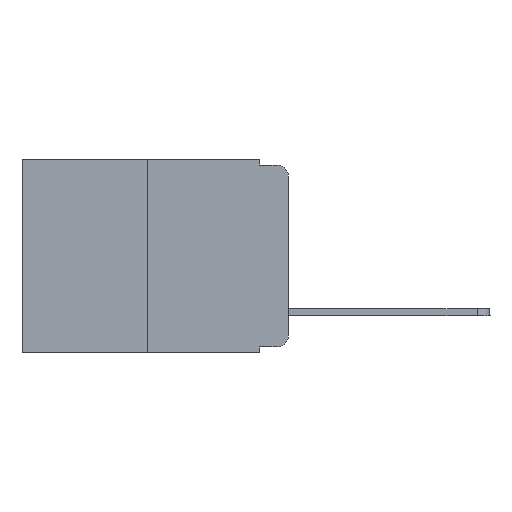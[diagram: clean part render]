
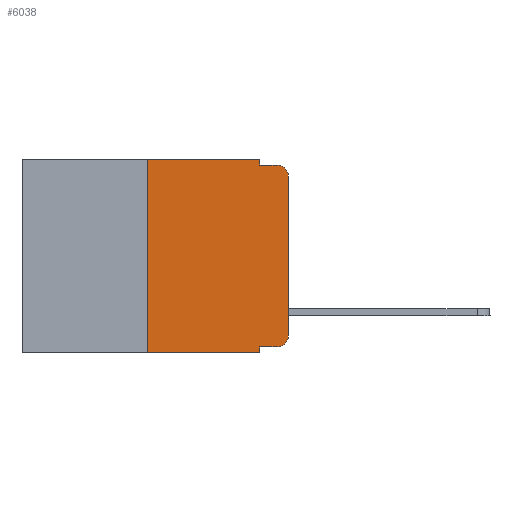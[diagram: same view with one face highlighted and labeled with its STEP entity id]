
A CAD part, left-side view. The second image highlights one B-rep face of the part: STEP entity #6038.
In plain terms, the highlighted planar face has unit normal (-1, 0, 0).
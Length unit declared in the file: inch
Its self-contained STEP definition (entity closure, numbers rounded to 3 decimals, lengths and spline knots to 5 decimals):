
#55 = LINE ( 'NONE', #207, #665 ) ;
#207 = CARTESIAN_POINT ( 'NONE',  ( 0., 0.051, 0. ) ) ;
#636 = CARTESIAN_POINT ( 'NONE',  ( 0., 0.25, 0. ) ) ;
#665 = VECTOR ( 'NONE', #2945, 39.37008 ) ;
#718 = DIRECTION ( 'NONE',  ( 0., 0., -1. ) ) ;
#817 = FACE_OUTER_BOUND ( 'NONE', #9570, .T. ) ;
#1017 = LINE ( 'NONE', #8204, #3437 ) ;
#1083 = VERTEX_POINT ( 'NONE', #6761 ) ;
#1377 = VECTOR ( 'NONE', #4258, 39.37008 ) ;
#1836 = DIRECTION ( 'NONE',  ( 0., 0., 1. ) ) ;
#1902 = DIRECTION ( 'NONE',  ( -1., 0., 0. ) ) ;
#1961 = EDGE_CURVE ( 'NONE', #9466, #3593, #12569, .T. ) ;
#2241 = ORIENTED_EDGE ( 'NONE', *, *, #13713, .T. ) ;
#2473 = EDGE_CURVE ( 'NONE', #8637, #9645, #10132, .T. ) ;
#2530 = CARTESIAN_POINT ( 'NONE',  ( 0., 0.051, -0.333 ) ) ;
#2765 = LINE ( 'NONE', #5359, #1377 ) ;
#2816 = CARTESIAN_POINT ( 'NONE',  ( 0., 0., -0.313 ) ) ;
#2838 = DIRECTION ( 'NONE',  ( 0., -1., 0. ) ) ;
#2945 = DIRECTION ( 'NONE',  ( 0., 0., -1. ) ) ;
#3437 = VECTOR ( 'NONE', #1836, 39.37008 ) ;
#3593 = VERTEX_POINT ( 'NONE', #9325 ) ;
#3836 = DIRECTION ( 'NONE',  ( -1., 0., 0. ) ) ;
#3956 = CIRCLE ( 'NONE', #6671, 0.02 ) ;
#4243 = AXIS2_PLACEMENT_3D ( 'NONE', #8437, #15005, #7209 ) ;
#4258 = DIRECTION ( 'NONE',  ( 0., -1., 0. ) ) ;
#4588 = CARTESIAN_POINT ( 'NONE',  ( 0., 0.25, -0.343 ) ) ;
#4940 = CARTESIAN_POINT ( 'NONE',  ( 0., 0.473, 0. ) ) ;
#5207 = CARTESIAN_POINT ( 'NONE',  ( 0., 0.051, -0.01 ) ) ;
#5359 = CARTESIAN_POINT ( 'NONE',  ( 0., 0.473, -0.343 ) ) ;
#5781 = EDGE_CURVE ( 'NONE', #1083, #15690, #7838, .T. ) ;
#5980 = EDGE_CURVE ( 'NONE', #6681, #8637, #1017, .T. ) ;
#6038 = ADVANCED_FACE ( 'NONE', ( #817 ), #14897, .F. ) ;
#6141 = LINE ( 'NONE', #14799, #15183 ) ;
#6408 = ORIENTED_EDGE ( 'NONE', *, *, #5980, .F. ) ;
#6595 = CARTESIAN_POINT ( 'NONE',  ( 0., 0.051, -0.01 ) ) ;
#6671 = AXIS2_PLACEMENT_3D ( 'NONE', #10953, #3836, #16038 ) ;
#6681 = VERTEX_POINT ( 'NONE', #4588 ) ;
#6761 = CARTESIAN_POINT ( 'NONE',  ( 0., 0.051, -0.333 ) ) ;
#6829 = VECTOR ( 'NONE', #12803, 39.37008 ) ;
#6850 = CIRCLE ( 'NONE', #14846, 0.02 ) ;
#6898 = VERTEX_POINT ( 'NONE', #5207 ) ;
#7050 = CARTESIAN_POINT ( 'NONE',  ( 0., 0.02, -0.03 ) ) ;
#7209 = DIRECTION ( 'NONE',  ( 0., 0., -1. ) ) ;
#7406 = EDGE_CURVE ( 'NONE', #6681, #9851, #2765, .T. ) ;
#7838 = LINE ( 'NONE', #2530, #6829 ) ;
#7950 = VECTOR ( 'NONE', #15920, 39.37008 ) ;
#8204 = CARTESIAN_POINT ( 'NONE',  ( 0., 0.25, 0. ) ) ;
#8404 = EDGE_CURVE ( 'NONE', #1083, #9851, #6141, .T. ) ;
#8436 = ORIENTED_EDGE ( 'NONE', *, *, #11366, .F. ) ;
#8437 = CARTESIAN_POINT ( 'NONE',  ( 0., 0.473, 0. ) ) ;
#8637 = VERTEX_POINT ( 'NONE', #636 ) ;
#8786 = ORIENTED_EDGE ( 'NONE', *, *, #7406, .T. ) ;
#8802 = ORIENTED_EDGE ( 'NONE', *, *, #5781, .T. ) ;
#8826 = DIRECTION ( 'NONE',  ( 0., -1., 0. ) ) ;
#9069 = ORIENTED_EDGE ( 'NONE', *, *, #11413, .F. ) ;
#9325 = CARTESIAN_POINT ( 'NONE',  ( 0., 0., -0.03 ) ) ;
#9411 = CARTESIAN_POINT ( 'NONE',  ( 0., 0., 0. ) ) ;
#9466 = VERTEX_POINT ( 'NONE', #2816 ) ;
#9570 = EDGE_LOOP ( 'NONE', ( #13248, #10444, #8436, #9069, #11517, #6408, #8786, #12966, #8802, #2241 ) ) ;
#9645 = VERTEX_POINT ( 'NONE', #11063 ) ;
#9683 = DIRECTION ( 'NONE',  ( 0., 0., -1. ) ) ;
#9851 = VERTEX_POINT ( 'NONE', #16337 ) ;
#9894 = CARTESIAN_POINT ( 'NONE',  ( 0., 0.02, -0.333 ) ) ;
#10132 = LINE ( 'NONE', #4940, #16182 ) ;
#10444 = ORIENTED_EDGE ( 'NONE', *, *, #12144, .T. ) ;
#10953 = CARTESIAN_POINT ( 'NONE',  ( 0., 0.02, -0.313 ) ) ;
#11063 = CARTESIAN_POINT ( 'NONE',  ( 0., 0.051, 0. ) ) ;
#11300 = VERTEX_POINT ( 'NONE', #15998 ) ;
#11366 = EDGE_CURVE ( 'NONE', #6898, #11300, #16326, .T. ) ;
#11413 = EDGE_CURVE ( 'NONE', #9645, #6898, #55, .T. ) ;
#11517 = ORIENTED_EDGE ( 'NONE', *, *, #2473, .F. ) ;
#12144 = EDGE_CURVE ( 'NONE', #3593, #11300, #6850, .T. ) ;
#12569 = LINE ( 'NONE', #9411, #7950 ) ;
#12803 = DIRECTION ( 'NONE',  ( 0., -1., 0. ) ) ;
#12890 = VECTOR ( 'NONE', #2838, 39.37008 ) ;
#12966 = ORIENTED_EDGE ( 'NONE', *, *, #8404, .F. ) ;
#13248 = ORIENTED_EDGE ( 'NONE', *, *, #1961, .T. ) ;
#13713 = EDGE_CURVE ( 'NONE', #15690, #9466, #3956, .T. ) ;
#14799 = CARTESIAN_POINT ( 'NONE',  ( 0., 0.051, 0. ) ) ;
#14846 = AXIS2_PLACEMENT_3D ( 'NONE', #7050, #1902, #9683 ) ;
#14897 = PLANE ( 'NONE',  #4243 ) ;
#15005 = DIRECTION ( 'NONE',  ( 1., 0., 0. ) ) ;
#15183 = VECTOR ( 'NONE', #718, 39.37008 ) ;
#15690 = VERTEX_POINT ( 'NONE', #9894 ) ;
#15920 = DIRECTION ( 'NONE',  ( 0., 0., 1. ) ) ;
#15998 = CARTESIAN_POINT ( 'NONE',  ( 0., 0.02, -0.01 ) ) ;
#16038 = DIRECTION ( 'NONE',  ( 0., 0., -1. ) ) ;
#16182 = VECTOR ( 'NONE', #8826, 39.37008 ) ;
#16326 = LINE ( 'NONE', #6595, #12890 ) ;
#16337 = CARTESIAN_POINT ( 'NONE',  ( 0., 0.051, -0.343 ) ) ;
